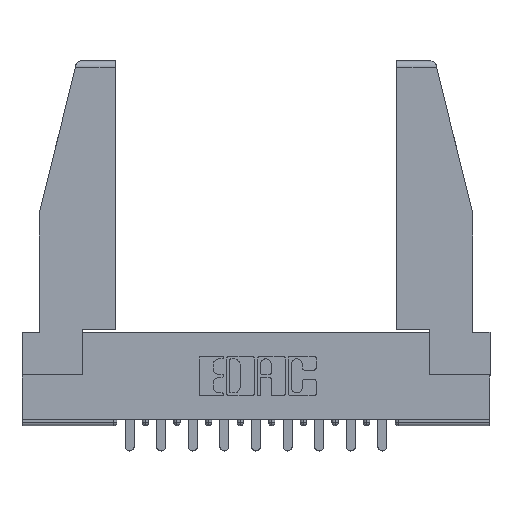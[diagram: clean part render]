
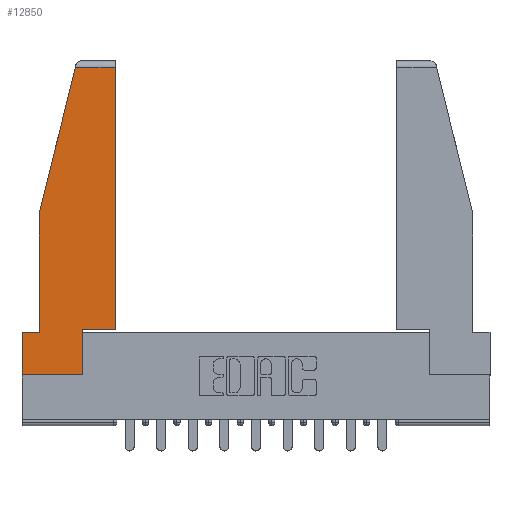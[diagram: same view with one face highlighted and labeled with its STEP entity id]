
A CAD part, top view. The second image highlights one B-rep face of the part: STEP entity #12850.
In plain terms, the highlighted planar face has unit normal (0, 0, 1).
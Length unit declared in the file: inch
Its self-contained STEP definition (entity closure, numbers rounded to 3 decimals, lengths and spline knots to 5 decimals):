
#100 = CARTESIAN_POINT ( 'NONE',  ( 0.271, 1.55, 0. ) ) ;
#726 = VECTOR ( 'NONE', #7624, 39.37008 ) ;
#751 = LINE ( 'NONE', #8348, #14369 ) ;
#792 = CARTESIAN_POINT ( 'NONE',  ( 0., 0., 0. ) ) ;
#881 = DIRECTION ( 'NONE',  ( 1., 0., 0. ) ) ;
#893 = LINE ( 'NONE', #100, #726 ) ;
#1779 = CARTESIAN_POINT ( 'NONE',  ( 0.297, 0.223, 0. ) ) ;
#1796 = ORIENTED_EDGE ( 'NONE', *, *, #5727, .T. ) ;
#1828 = ORIENTED_EDGE ( 'NONE', *, *, #14689, .T. ) ;
#1845 = LINE ( 'NONE', #792, #3754 ) ;
#1917 = LINE ( 'NONE', #12170, #11956 ) ;
#2329 = EDGE_CURVE ( 'NONE', #12185, #9989, #7190, .T. ) ;
#2543 = CARTESIAN_POINT ( 'NONE',  ( 0.086, 0.21, 0. ) ) ;
#2592 = VECTOR ( 'NONE', #13135, 39.37008 ) ;
#2791 = ORIENTED_EDGE ( 'NONE', *, *, #5855, .T. ) ;
#3478 = DIRECTION ( 'NONE',  ( 0., 1., 0. ) ) ;
#3754 = VECTOR ( 'NONE', #881, 39.37008 ) ;
#4491 = CARTESIAN_POINT ( 'NONE',  ( 0.461, 0.223, 0. ) ) ;
#4643 = EDGE_CURVE ( 'NONE', #11227, #13443, #751, .T. ) ;
#4856 = DIRECTION ( 'NONE',  ( 0., 0., 1. ) ) ;
#5407 = VECTOR ( 'NONE', #3478, 39.37008 ) ;
#5727 = EDGE_CURVE ( 'NONE', #13443, #8520, #1917, .T. ) ;
#5855 = EDGE_CURVE ( 'NONE', #8300, #14257, #9087, .T. ) ;
#5874 = LINE ( 'NONE', #6887, #2592 ) ;
#5930 = LINE ( 'NONE', #1779, #13511 ) ;
#6064 = DIRECTION ( 'NONE',  ( -1., 0., 0. ) ) ;
#6429 = VECTOR ( 'NONE', #6981, 39.37008 ) ;
#6628 = CARTESIAN_POINT ( 'NONE',  ( 0.297, 0.223, 0. ) ) ;
#6702 = FACE_OUTER_BOUND ( 'NONE', #11521, .T. ) ;
#6768 = ORIENTED_EDGE ( 'NONE', *, *, #11225, .T. ) ;
#6799 = EDGE_CURVE ( 'NONE', #14257, #12185, #5930, .T. ) ;
#6887 = CARTESIAN_POINT ( 'NONE',  ( 0., 0.21, 0. ) ) ;
#6981 = DIRECTION ( 'NONE',  ( 0., 1., 0. ) ) ;
#7190 = LINE ( 'NONE', #4491, #6429 ) ;
#7624 = DIRECTION ( 'NONE',  ( -0.239, -0.971, 0. ) ) ;
#8038 = ORIENTED_EDGE ( 'NONE', *, *, #8333, .T. ) ;
#8239 = ORIENTED_EDGE ( 'NONE', *, *, #6799, .T. ) ;
#8300 = VERTEX_POINT ( 'NONE', #8829 ) ;
#8333 = EDGE_CURVE ( 'NONE', #11581, #8300, #1845, .T. ) ;
#8348 = CARTESIAN_POINT ( 'NONE',  ( 0.086, 0.8, 0. ) ) ;
#8387 = ORIENTED_EDGE ( 'NONE', *, *, #2329, .T. ) ;
#8520 = VERTEX_POINT ( 'NONE', #15548 ) ;
#8617 = EDGE_CURVE ( 'NONE', #8520, #11581, #5874, .T. ) ;
#8755 = VECTOR ( 'NONE', #6064, 39.37008 ) ;
#8829 = CARTESIAN_POINT ( 'NONE',  ( 0.297, 0., 0. ) ) ;
#8973 = ORIENTED_EDGE ( 'NONE', *, *, #8617, .T. ) ;
#9087 = LINE ( 'NONE', #14503, #5407 ) ;
#9854 = CARTESIAN_POINT ( 'NONE',  ( 0., 1.52, 0. ) ) ;
#9989 = VERTEX_POINT ( 'NONE', #12375 ) ;
#10859 = VERTEX_POINT ( 'NONE', #11869 ) ;
#10965 = CARTESIAN_POINT ( 'NONE',  ( 0.461, 0.223, 0. ) ) ;
#11225 = EDGE_CURVE ( 'NONE', #10859, #11227, #893, .T. ) ;
#11227 = VERTEX_POINT ( 'NONE', #11540 ) ;
#11521 = EDGE_LOOP ( 'NONE', ( #8387, #1828, #6768, #13239, #1796, #8973, #8038, #2791, #8239 ) ) ;
#11540 = CARTESIAN_POINT ( 'NONE',  ( 0.086, 0.8, 0. ) ) ;
#11581 = VERTEX_POINT ( 'NONE', #15643 ) ;
#11869 = CARTESIAN_POINT ( 'NONE',  ( 0.2636, 1.52, 0. ) ) ;
#11956 = VECTOR ( 'NONE', #15904, 39.37008 ) ;
#12040 = LINE ( 'NONE', #9854, #8755 ) ;
#12170 = CARTESIAN_POINT ( 'NONE',  ( 0., 0.21, 0. ) ) ;
#12185 = VERTEX_POINT ( 'NONE', #10965 ) ;
#12375 = CARTESIAN_POINT ( 'NONE',  ( 0.461, 1.52, 0. ) ) ;
#12763 = AXIS2_PLACEMENT_3D ( 'NONE', #13238, #4856, #13509 ) ;
#12850 = ADVANCED_FACE ( 'NONE', ( #6702 ), #14658, .T. ) ;
#13135 = DIRECTION ( 'NONE',  ( 0., -1., 0. ) ) ;
#13238 = CARTESIAN_POINT ( 'NONE',  ( 0., 0., 0. ) ) ;
#13239 = ORIENTED_EDGE ( 'NONE', *, *, #4643, .T. ) ;
#13334 = DIRECTION ( 'NONE',  ( 0., -1., 0. ) ) ;
#13443 = VERTEX_POINT ( 'NONE', #2543 ) ;
#13509 = DIRECTION ( 'NONE',  ( 1., 0., 0. ) ) ;
#13511 = VECTOR ( 'NONE', #15399, 39.37008 ) ;
#14257 = VERTEX_POINT ( 'NONE', #6628 ) ;
#14369 = VECTOR ( 'NONE', #13334, 39.37008 ) ;
#14503 = CARTESIAN_POINT ( 'NONE',  ( 0.297, 0., 0. ) ) ;
#14658 = PLANE ( 'NONE',  #12763 ) ;
#14689 = EDGE_CURVE ( 'NONE', #9989, #10859, #12040, .T. ) ;
#15399 = DIRECTION ( 'NONE',  ( 1., 0., 0. ) ) ;
#15548 = CARTESIAN_POINT ( 'NONE',  ( 0., 0.21, 0. ) ) ;
#15643 = CARTESIAN_POINT ( 'NONE',  ( 0., 0., 0. ) ) ;
#15904 = DIRECTION ( 'NONE',  ( -1., 0., 0. ) ) ;
